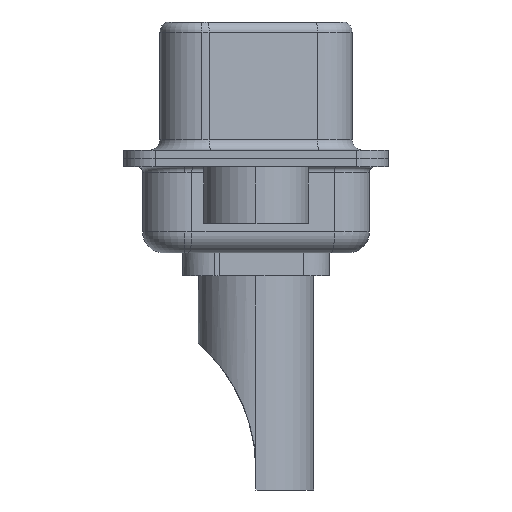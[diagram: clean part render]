
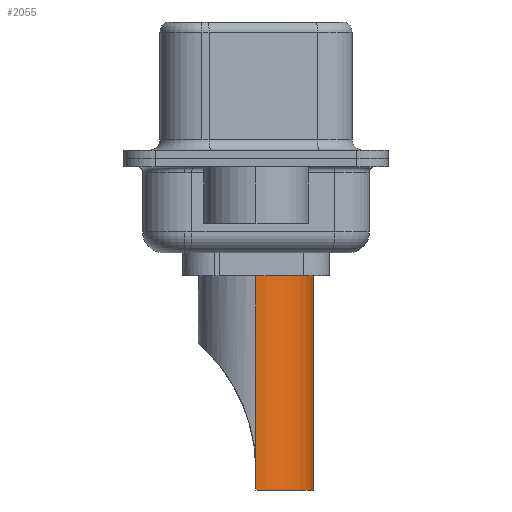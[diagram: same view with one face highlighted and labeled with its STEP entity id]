
A CAD part, left-side view. The second image highlights one B-rep face of the part: STEP entity #2055.
In plain terms, the highlighted cylindrical face has radius 2.75 mm (diameter 5.5 mm), a partial arc.
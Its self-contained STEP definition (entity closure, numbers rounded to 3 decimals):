
#14 = DIRECTION ( 'NONE',  ( 1., 0., 0. ) ) ;
#847 = FACE_OUTER_BOUND ( 'NONE', #10630, .T. ) ;
#883 = ORIENTED_EDGE ( 'NONE', *, *, #1564, .T. ) ;
#1231 = LINE ( 'NONE', #13382, #14240 ) ;
#1564 = EDGE_CURVE ( 'NONE', #12804, #8297, #7932, .T. ) ;
#1886 = ORIENTED_EDGE ( 'NONE', *, *, #13851, .F. ) ;
#1914 = LINE ( 'NONE', #9410, #4780 ) ;
#1944 = CARTESIAN_POINT ( 'NONE',  ( 2.75, 0., -7.764 ) ) ;
#2055 = ADVANCED_FACE ( 'NONE', ( #847 ), #3708, .T. ) ;
#2512 = CARTESIAN_POINT ( 'NONE',  ( 0., 0., -8.7 ) ) ;
#3017 = VERTEX_POINT ( 'NONE', #12939 ) ;
#3708 = CYLINDRICAL_SURFACE ( 'NONE', #9053, 2.75 ) ;
#3777 = LINE ( 'NONE', #13671, #12782 ) ;
#4410 = AXIS2_PLACEMENT_3D ( 'NONE', #6110, #6010, #5494 ) ;
#4464 = CARTESIAN_POINT ( 'NONE',  ( 2.75, 0., -8.7 ) ) ;
#4780 = VECTOR ( 'NONE', #14835, 1000. ) ;
#5494 = DIRECTION ( 'NONE',  ( 1., 0., 0. ) ) ;
#6010 = DIRECTION ( 'NONE',  ( 0., 0., 1. ) ) ;
#6034 = DIRECTION ( 'NONE',  ( 0., 0., 1. ) ) ;
#6110 = CARTESIAN_POINT ( 'NONE',  ( 0., 0., 1.5 ) ) ;
#6783 = CARTESIAN_POINT ( 'NONE',  ( 2.75, 0., 1.5 ) ) ;
#7383 = EDGE_CURVE ( 'NONE', #3017, #12804, #1914, .T. ) ;
#7423 = DIRECTION ( 'NONE',  ( 0., 0., -1. ) ) ;
#7932 = CIRCLE ( 'NONE', #15442, 2.75 ) ;
#8196 = ORIENTED_EDGE ( 'NONE', *, *, #12511, .T. ) ;
#8297 = VERTEX_POINT ( 'NONE', #4464 ) ;
#8701 = EDGE_CURVE ( 'NONE', #3017, #10370, #3777, .T. ) ;
#9053 = AXIS2_PLACEMENT_3D ( 'NONE', #11560, #9411, #14 ) ;
#9074 = CARTESIAN_POINT ( 'NONE',  ( -2.75, 0., -8.7 ) ) ;
#9303 = ORIENTED_EDGE ( 'NONE', *, *, #7383, .T. ) ;
#9410 = CARTESIAN_POINT ( 'NONE',  ( -2.75, 0., -8.7 ) ) ;
#9411 = DIRECTION ( 'NONE',  ( 0., 0., 1. ) ) ;
#9575 = VERTEX_POINT ( 'NONE', #1944 ) ;
#9608 = DIRECTION ( 'NONE',  ( 0., 0., 1. ) ) ;
#9780 = VECTOR ( 'NONE', #7423, 1000. ) ;
#9851 = CARTESIAN_POINT ( 'NONE',  ( 2.75, 0., -8.7 ) ) ;
#10017 = EDGE_CURVE ( 'NONE', #10370, #14143, #12540, .T. ) ;
#10370 = VERTEX_POINT ( 'NONE', #14525 ) ;
#10630 = EDGE_LOOP ( 'NONE', ( #11367, #9303, #883, #1886, #8196, #12361 ) ) ;
#11113 = DIRECTION ( 'NONE',  ( 1., 0., 0. ) ) ;
#11367 = ORIENTED_EDGE ( 'NONE', *, *, #8701, .F. ) ;
#11560 = CARTESIAN_POINT ( 'NONE',  ( 0., 0., 4.234 ) ) ;
#12361 = ORIENTED_EDGE ( 'NONE', *, *, #10017, .F. ) ;
#12511 = EDGE_CURVE ( 'NONE', #9575, #14143, #1231, .T. ) ;
#12540 = CIRCLE ( 'NONE', #4410, 2.75 ) ;
#12583 = DIRECTION ( 'NONE',  ( 0., 0., 1. ) ) ;
#12782 = VECTOR ( 'NONE', #9608, 1000. ) ;
#12804 = VERTEX_POINT ( 'NONE', #9074 ) ;
#12939 = CARTESIAN_POINT ( 'NONE',  ( -2.75, 0., -7.764 ) ) ;
#13382 = CARTESIAN_POINT ( 'NONE',  ( 2.75, 0., 4.234 ) ) ;
#13456 = LINE ( 'NONE', #9851, #9780 ) ;
#13671 = CARTESIAN_POINT ( 'NONE',  ( -2.75, 0., 4.234 ) ) ;
#13851 = EDGE_CURVE ( 'NONE', #9575, #8297, #13456, .T. ) ;
#14143 = VERTEX_POINT ( 'NONE', #6783 ) ;
#14240 = VECTOR ( 'NONE', #6034, 1000. ) ;
#14525 = CARTESIAN_POINT ( 'NONE',  ( -2.75, 0., 1.5 ) ) ;
#14835 = DIRECTION ( 'NONE',  ( 0., 0., -1. ) ) ;
#15442 = AXIS2_PLACEMENT_3D ( 'NONE', #2512, #12583, #11113 ) ;
